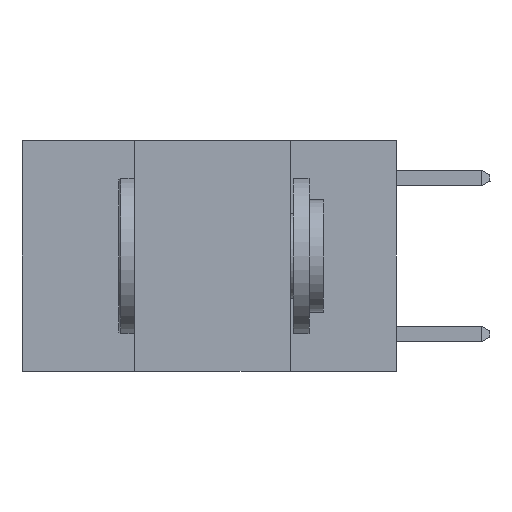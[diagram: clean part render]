
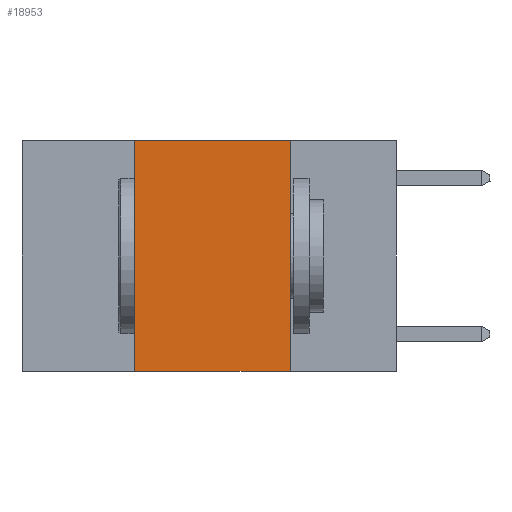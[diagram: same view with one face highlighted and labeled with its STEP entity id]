
A CAD part, left-side view. The second image highlights one B-rep face of the part: STEP entity #18953.
In plain terms, the highlighted planar face has unit normal (-1, 0, 0).
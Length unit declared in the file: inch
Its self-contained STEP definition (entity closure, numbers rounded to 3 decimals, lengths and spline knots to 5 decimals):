
#259 = AXIS2_PLACEMENT_3D ( 'NONE', #23058, #19581, #8716 ) ;
#735 = VERTEX_POINT ( 'NONE', #3792 ) ;
#1464 = LINE ( 'NONE', #13032, #8688 ) ;
#1642 = CARTESIAN_POINT ( 'NONE',  ( 0., 0.17, 0. ) ) ;
#1728 = DIRECTION ( 'NONE',  ( 0., -1., 0. ) ) ;
#2223 = DIRECTION ( 'NONE',  ( 0., 0., 1. ) ) ;
#2700 = VERTEX_POINT ( 'NONE', #1642 ) ;
#3792 = CARTESIAN_POINT ( 'NONE',  ( 0., 0.42, -0.37 ) ) ;
#4338 = EDGE_CURVE ( 'NONE', #11931, #2700, #19074, .T. ) ;
#4365 = VERTEX_POINT ( 'NONE', #21760 ) ;
#7720 = EDGE_CURVE ( 'NONE', #735, #11931, #21725, .T. ) ;
#8688 = VECTOR ( 'NONE', #9318, 39.37008 ) ;
#8716 = DIRECTION ( 'NONE',  ( 0., 0., -1. ) ) ;
#8891 = DIRECTION ( 'NONE',  ( 0., 0., -1. ) ) ;
#8940 = EDGE_CURVE ( 'NONE', #735, #4365, #1464, .T. ) ;
#9318 = DIRECTION ( 'NONE',  ( 0., -1., 0. ) ) ;
#10166 = EDGE_CURVE ( 'NONE', #2700, #4365, #18268, .T. ) ;
#10455 = VECTOR ( 'NONE', #2223, 39.37008 ) ;
#11931 = VERTEX_POINT ( 'NONE', #17293 ) ;
#13032 = CARTESIAN_POINT ( 'NONE',  ( 0., 0.6, -0.37 ) ) ;
#13249 = CARTESIAN_POINT ( 'NONE',  ( 0., 0.42, 0. ) ) ;
#14626 = FACE_OUTER_BOUND ( 'NONE', #16083, .T. ) ;
#15939 = PLANE ( 'NONE',  #259 ) ;
#16083 = EDGE_LOOP ( 'NONE', ( #20486, #20552, #21123, #21140 ) ) ;
#16369 = CARTESIAN_POINT ( 'NONE',  ( 0., 0.6, 0. ) ) ;
#17293 = CARTESIAN_POINT ( 'NONE',  ( 0., 0.42, 0. ) ) ;
#18268 = LINE ( 'NONE', #23311, #22464 ) ;
#18499 = VECTOR ( 'NONE', #1728, 39.37008 ) ;
#18953 = ADVANCED_FACE ( 'NONE', ( #14626 ), #15939, .F. ) ;
#19074 = LINE ( 'NONE', #16369, #18499 ) ;
#19581 = DIRECTION ( 'NONE',  ( 1., 0., 0. ) ) ;
#20486 = ORIENTED_EDGE ( 'NONE', *, *, #10166, .F. ) ;
#20552 = ORIENTED_EDGE ( 'NONE', *, *, #4338, .F. ) ;
#21123 = ORIENTED_EDGE ( 'NONE', *, *, #7720, .F. ) ;
#21140 = ORIENTED_EDGE ( 'NONE', *, *, #8940, .T. ) ;
#21725 = LINE ( 'NONE', #13249, #10455 ) ;
#21760 = CARTESIAN_POINT ( 'NONE',  ( 0., 0.17, -0.37 ) ) ;
#22464 = VECTOR ( 'NONE', #8891, 39.37008 ) ;
#23058 = CARTESIAN_POINT ( 'NONE',  ( 0., 0.6, 0. ) ) ;
#23311 = CARTESIAN_POINT ( 'NONE',  ( 0., 0.17, 0. ) ) ;
